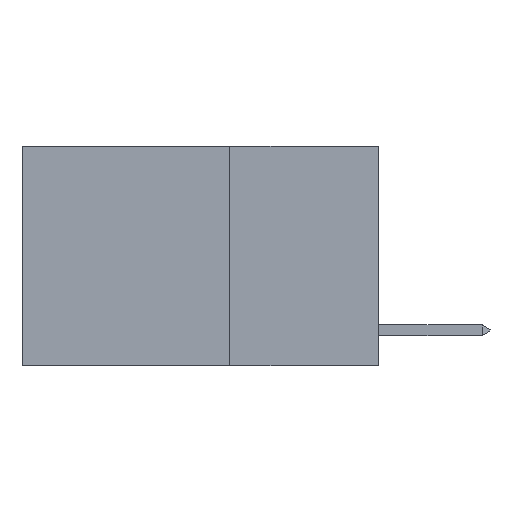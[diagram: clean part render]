
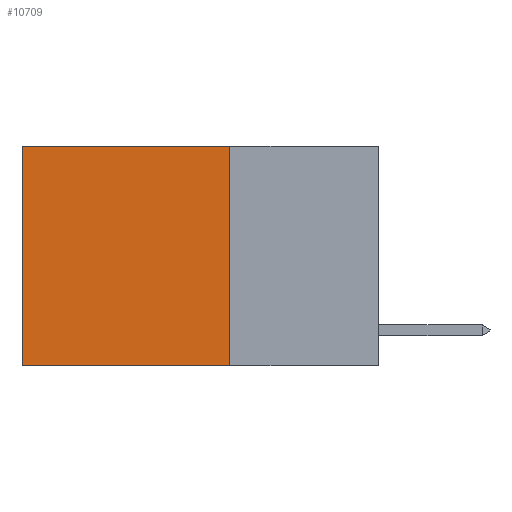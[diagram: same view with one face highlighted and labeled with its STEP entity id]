
A CAD part, left-side view. The second image highlights one B-rep face of the part: STEP entity #10709.
In plain terms, the highlighted planar face has unit normal (-1, 0, 0).
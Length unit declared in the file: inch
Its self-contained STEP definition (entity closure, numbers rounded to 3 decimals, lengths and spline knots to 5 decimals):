
#1680 = VECTOR ( 'NONE', #16234, 39.37008 ) ;
#1884 = EDGE_CURVE ( 'NONE', #8557, #10546, #10329, .T. ) ;
#1987 = DIRECTION ( 'NONE',  ( 1., 0., 0. ) ) ;
#2026 = VERTEX_POINT ( 'NONE', #5117 ) ;
#2091 = EDGE_CURVE ( 'NONE', #8328, #2026, #18407, .T. ) ;
#3828 = ORIENTED_EDGE ( 'NONE', *, *, #11933, .F. ) ;
#5117 = CARTESIAN_POINT ( 'NONE',  ( 0.2625, 0.6, -0.37 ) ) ;
#5682 = CARTESIAN_POINT ( 'NONE',  ( 0.2625, 0.25, 0. ) ) ;
#5785 = ORIENTED_EDGE ( 'NONE', *, *, #1884, .T. ) ;
#6582 = CARTESIAN_POINT ( 'NONE',  ( 0.2625, 0.25, -0.37 ) ) ;
#7875 = CARTESIAN_POINT ( 'NONE',  ( 0.2625, 0.6, 0. ) ) ;
#8098 = CARTESIAN_POINT ( 'NONE',  ( 0.2625, 0.25, 0. ) ) ;
#8328 = VERTEX_POINT ( 'NONE', #6582 ) ;
#8557 = VERTEX_POINT ( 'NONE', #5682 ) ;
#9671 = EDGE_LOOP ( 'NONE', ( #19676, #16998, #3828, #5785 ) ) ;
#10329 = LINE ( 'NONE', #11373, #14500 ) ;
#10546 = VERTEX_POINT ( 'NONE', #7875 ) ;
#10579 = AXIS2_PLACEMENT_3D ( 'NONE', #16126, #1987, #13031 ) ;
#10709 = ADVANCED_FACE ( 'NONE', ( #17418 ), #11457, .F. ) ;
#11373 = CARTESIAN_POINT ( 'NONE',  ( 0.2625, 0.25, 0. ) ) ;
#11457 = PLANE ( 'NONE',  #10579 ) ;
#11638 = DIRECTION ( 'NONE',  ( 0., 1., 0. ) ) ;
#11933 = EDGE_CURVE ( 'NONE', #8557, #8328, #19294, .T. ) ;
#12468 = VECTOR ( 'NONE', #12849, 39.37008 ) ;
#12849 = DIRECTION ( 'NONE',  ( 0., 0., -1. ) ) ;
#13031 = DIRECTION ( 'NONE',  ( 0., 0., -1. ) ) ;
#13116 = DIRECTION ( 'NONE',  ( 0., 0., -1. ) ) ;
#14500 = VECTOR ( 'NONE', #11638, 39.37008 ) ;
#14688 = CARTESIAN_POINT ( 'NONE',  ( 0.2625, 0.6, 0. ) ) ;
#14721 = LINE ( 'NONE', #14688, #18395 ) ;
#14875 = EDGE_CURVE ( 'NONE', #10546, #2026, #14721, .T. ) ;
#16126 = CARTESIAN_POINT ( 'NONE',  ( 0.2625, 0.25, 0. ) ) ;
#16234 = DIRECTION ( 'NONE',  ( 0., 1., 0. ) ) ;
#16836 = CARTESIAN_POINT ( 'NONE',  ( 0.2625, 0.25, -0.37 ) ) ;
#16998 = ORIENTED_EDGE ( 'NONE', *, *, #2091, .F. ) ;
#17418 = FACE_OUTER_BOUND ( 'NONE', #9671, .T. ) ;
#18395 = VECTOR ( 'NONE', #13116, 39.37008 ) ;
#18407 = LINE ( 'NONE', #16836, #1680 ) ;
#19294 = LINE ( 'NONE', #8098, #12468 ) ;
#19676 = ORIENTED_EDGE ( 'NONE', *, *, #14875, .T. ) ;
